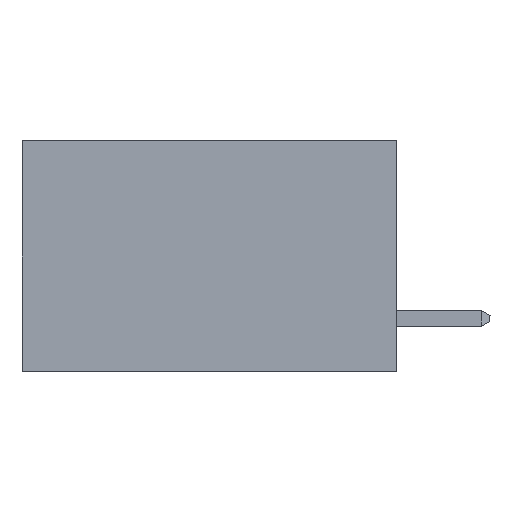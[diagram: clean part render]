
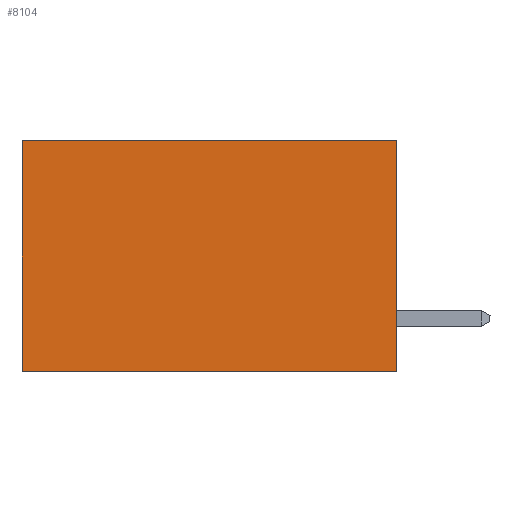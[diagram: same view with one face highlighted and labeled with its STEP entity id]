
A CAD part, left-side view. The second image highlights one B-rep face of the part: STEP entity #8104.
In plain terms, the highlighted planar face has unit normal (-1, 0, 0).
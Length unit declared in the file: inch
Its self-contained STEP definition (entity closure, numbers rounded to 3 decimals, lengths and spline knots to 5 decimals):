
#350 = CARTESIAN_POINT ( 'NONE',  ( 0.2615, 0., -0.37 ) ) ;
#1838 = EDGE_CURVE ( 'NONE', #18045, #11485, #3597, .T. ) ;
#1963 = VECTOR ( 'NONE', #9938, 39.37008 ) ;
#2105 = LINE ( 'NONE', #15526, #13378 ) ;
#3111 = AXIS2_PLACEMENT_3D ( 'NONE', #18212, #17963, #17944 ) ;
#3597 = LINE ( 'NONE', #13079, #6479 ) ;
#4132 = VERTEX_POINT ( 'NONE', #5468 ) ;
#4772 = ORIENTED_EDGE ( 'NONE', *, *, #13733, .T. ) ;
#5141 = ORIENTED_EDGE ( 'NONE', *, *, #7592, .F. ) ;
#5460 = ORIENTED_EDGE ( 'NONE', *, *, #1838, .F. ) ;
#5468 = CARTESIAN_POINT ( 'NONE',  ( 0.2615, 0.6, -0.37 ) ) ;
#6479 = VECTOR ( 'NONE', #10022, 39.37008 ) ;
#7478 = EDGE_LOOP ( 'NONE', ( #4772, #5141, #5460, #9809 ) ) ;
#7592 = EDGE_CURVE ( 'NONE', #11485, #4132, #9665, .T. ) ;
#8104 = ADVANCED_FACE ( 'NONE', ( #8471 ), #18122, .F. ) ;
#8396 = VERTEX_POINT ( 'NONE', #15170 ) ;
#8471 = FACE_OUTER_BOUND ( 'NONE', #7478, .T. ) ;
#9595 = CARTESIAN_POINT ( 'NONE',  ( 0.2615, 0.6, -0.37 ) ) ;
#9665 = LINE ( 'NONE', #10002, #1963 ) ;
#9809 = ORIENTED_EDGE ( 'NONE', *, *, #12911, .T. ) ;
#9938 = DIRECTION ( 'NONE',  ( 0., 1., 0. ) ) ;
#10002 = CARTESIAN_POINT ( 'NONE',  ( 0.2615, 0., -0.37 ) ) ;
#10022 = DIRECTION ( 'NONE',  ( 0., 0., -1. ) ) ;
#11485 = VERTEX_POINT ( 'NONE', #350 ) ;
#11528 = DIRECTION ( 'NONE',  ( 0., 0., -1. ) ) ;
#12911 = EDGE_CURVE ( 'NONE', #18045, #8396, #2105, .T. ) ;
#13079 = CARTESIAN_POINT ( 'NONE',  ( 0.2615, 0., -0.37 ) ) ;
#13378 = VECTOR ( 'NONE', #15668, 39.37008 ) ;
#13733 = EDGE_CURVE ( 'NONE', #8396, #4132, #17882, .T. ) ;
#14107 = CARTESIAN_POINT ( 'NONE',  ( 0.2615, 0., 0. ) ) ;
#14229 = VECTOR ( 'NONE', #11528, 39.37008 ) ;
#15170 = CARTESIAN_POINT ( 'NONE',  ( 0.2615, 0.6, 0. ) ) ;
#15526 = CARTESIAN_POINT ( 'NONE',  ( 0.2615, 0., 0. ) ) ;
#15668 = DIRECTION ( 'NONE',  ( 0., 1., 0. ) ) ;
#17882 = LINE ( 'NONE', #9595, #14229 ) ;
#17944 = DIRECTION ( 'NONE',  ( 0., 0., -1. ) ) ;
#17963 = DIRECTION ( 'NONE',  ( 1., 0., 0. ) ) ;
#18045 = VERTEX_POINT ( 'NONE', #14107 ) ;
#18122 = PLANE ( 'NONE',  #3111 ) ;
#18212 = CARTESIAN_POINT ( 'NONE',  ( 0.2615, 0., -0.37 ) ) ;
